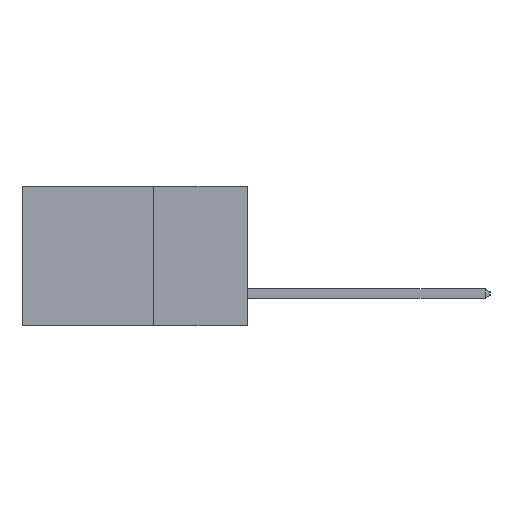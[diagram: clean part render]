
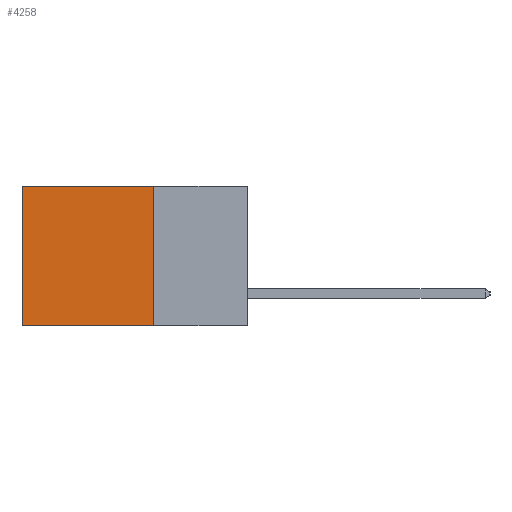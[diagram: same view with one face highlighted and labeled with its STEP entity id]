
A CAD part, left-side view. The second image highlights one B-rep face of the part: STEP entity #4258.
In plain terms, the highlighted planar face has unit normal (-1, 0, 0).
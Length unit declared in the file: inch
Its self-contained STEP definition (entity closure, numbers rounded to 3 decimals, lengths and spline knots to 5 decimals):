
#460 = CARTESIAN_POINT ( 'NONE',  ( 0.2615, 0.25, -0.37 ) ) ;
#563 = EDGE_LOOP ( 'NONE', ( #2422, #2832, #2567, #2850 ) ) ;
#653 = EDGE_CURVE ( 'NONE', #2248, #5471, #856, .T. ) ;
#856 = LINE ( 'NONE', #3319, #5218 ) ;
#1176 = VECTOR ( 'NONE', #3656, 39.37008 ) ;
#1671 = LINE ( 'NONE', #2646, #3485 ) ;
#1690 = DIRECTION ( 'NONE',  ( 0., 0., -1. ) ) ;
#1691 = DIRECTION ( 'NONE',  ( 1., 0., 0. ) ) ;
#2248 = VERTEX_POINT ( 'NONE', #9075 ) ;
#2422 = ORIENTED_EDGE ( 'NONE', *, *, #7958, .T. ) ;
#2567 = ORIENTED_EDGE ( 'NONE', *, *, #8967, .F. ) ;
#2646 = CARTESIAN_POINT ( 'NONE',  ( 0.2615, 0.25, -0.37 ) ) ;
#2832 = ORIENTED_EDGE ( 'NONE', *, *, #9361, .F. ) ;
#2850 = ORIENTED_EDGE ( 'NONE', *, *, #653, .T. ) ;
#2894 = CARTESIAN_POINT ( 'NONE',  ( 0.2615, 0.25, -0.37 ) ) ;
#3319 = CARTESIAN_POINT ( 'NONE',  ( 0.2615, 0.25, 0. ) ) ;
#3485 = VECTOR ( 'NONE', #4946, 39.37008 ) ;
#3509 = VECTOR ( 'NONE', #7575, 39.37008 ) ;
#3530 = CARTESIAN_POINT ( 'NONE',  ( 0.2615, 0.25, -0.37 ) ) ;
#3656 = DIRECTION ( 'NONE',  ( 0., 0., -1. ) ) ;
#3712 = VERTEX_POINT ( 'NONE', #460 ) ;
#3748 = LINE ( 'NONE', #3862, #3509 ) ;
#3842 = PLANE ( 'NONE',  #4294 ) ;
#3862 = CARTESIAN_POINT ( 'NONE',  ( 0.2615, 0.6, -0.37 ) ) ;
#3900 = CARTESIAN_POINT ( 'NONE',  ( 0.2615, 0.6, 0. ) ) ;
#4258 = ADVANCED_FACE ( 'NONE', ( #6413 ), #3842, .F. ) ;
#4294 = AXIS2_PLACEMENT_3D ( 'NONE', #3530, #1691, #1690 ) ;
#4466 = DIRECTION ( 'NONE',  ( 0., 1., 0. ) ) ;
#4849 = CARTESIAN_POINT ( 'NONE',  ( 0.2615, 0.6, -0.37 ) ) ;
#4946 = DIRECTION ( 'NONE',  ( 0., 1., 0. ) ) ;
#5218 = VECTOR ( 'NONE', #4466, 39.37008 ) ;
#5284 = LINE ( 'NONE', #2894, #1176 ) ;
#5471 = VERTEX_POINT ( 'NONE', #3900 ) ;
#6413 = FACE_OUTER_BOUND ( 'NONE', #563, .T. ) ;
#7575 = DIRECTION ( 'NONE',  ( 0., 0., -1. ) ) ;
#7958 = EDGE_CURVE ( 'NONE', #5471, #9285, #3748, .T. ) ;
#8967 = EDGE_CURVE ( 'NONE', #2248, #3712, #5284, .T. ) ;
#9075 = CARTESIAN_POINT ( 'NONE',  ( 0.2615, 0.25, 0. ) ) ;
#9285 = VERTEX_POINT ( 'NONE', #4849 ) ;
#9361 = EDGE_CURVE ( 'NONE', #3712, #9285, #1671, .T. ) ;
